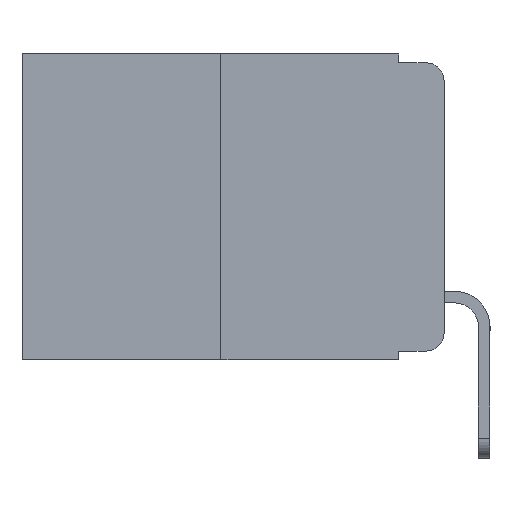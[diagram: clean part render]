
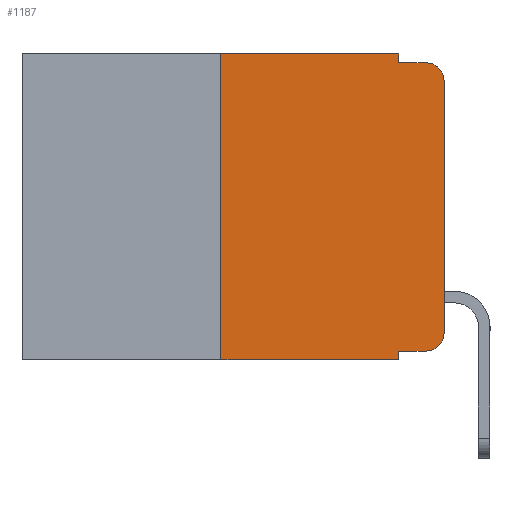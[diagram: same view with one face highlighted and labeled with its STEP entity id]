
A CAD part, left-side view. The second image highlights one B-rep face of the part: STEP entity #1187.
In plain terms, the highlighted planar face has unit normal (-1, 0, 0).
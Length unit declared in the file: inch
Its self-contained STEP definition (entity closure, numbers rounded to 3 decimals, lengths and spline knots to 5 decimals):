
#243 = ORIENTED_EDGE ( 'NONE', *, *, #24246, .T. ) ;
#959 = VERTEX_POINT ( 'NONE', #16289 ) ;
#1187 = ADVANCED_FACE ( 'NONE', ( #11730 ), #17278, .F. ) ;
#1302 = DIRECTION ( 'NONE',  ( 0., 0., -1. ) ) ;
#1364 = CARTESIAN_POINT ( 'NONE',  ( 0., 0., 0. ) ) ;
#1775 = CARTESIAN_POINT ( 'NONE',  ( 0., 0.051, 0. ) ) ;
#1872 = DIRECTION ( 'NONE',  ( 0., 0., -1. ) ) ;
#2029 = CARTESIAN_POINT ( 'NONE',  ( 0., 0.473, 0. ) ) ;
#2393 = ORIENTED_EDGE ( 'NONE', *, *, #10809, .F. ) ;
#2582 = ORIENTED_EDGE ( 'NONE', *, *, #19447, .F. ) ;
#2783 = LINE ( 'NONE', #19544, #12855 ) ;
#2857 = ORIENTED_EDGE ( 'NONE', *, *, #24707, .F. ) ;
#2881 = EDGE_CURVE ( 'NONE', #23649, #20933, #2783, .T. ) ;
#3012 = VERTEX_POINT ( 'NONE', #13358 ) ;
#3714 = VERTEX_POINT ( 'NONE', #15313 ) ;
#3827 = CARTESIAN_POINT ( 'NONE',  ( 0., 0.051, -0.333 ) ) ;
#4040 = CARTESIAN_POINT ( 'NONE',  ( 0., 0.051, -0.333 ) ) ;
#4198 = AXIS2_PLACEMENT_3D ( 'NONE', #2029, #18192, #18045 ) ;
#5019 = EDGE_CURVE ( 'NONE', #3714, #23166, #5313, .T. ) ;
#5313 = LINE ( 'NONE', #14935, #11199 ) ;
#6075 = EDGE_CURVE ( 'NONE', #959, #22323, #8268, .T. ) ;
#6189 = VERTEX_POINT ( 'NONE', #16887 ) ;
#6404 = VERTEX_POINT ( 'NONE', #3827 ) ;
#6521 = LINE ( 'NONE', #4040, #21585 ) ;
#6672 = CARTESIAN_POINT ( 'NONE',  ( 0., 0.051, 0. ) ) ;
#6964 = VERTEX_POINT ( 'NONE', #13438 ) ;
#7321 = AXIS2_PLACEMENT_3D ( 'NONE', #14525, #14499, #9034 ) ;
#7905 = ORIENTED_EDGE ( 'NONE', *, *, #24487, .T. ) ;
#8268 = CIRCLE ( 'NONE', #7321, 0.02 ) ;
#8710 = DIRECTION ( 'NONE',  ( 0., 0., -1. ) ) ;
#8722 = AXIS2_PLACEMENT_3D ( 'NONE', #24347, #13497, #1302 ) ;
#8977 = ORIENTED_EDGE ( 'NONE', *, *, #5019, .F. ) ;
#9034 = DIRECTION ( 'NONE',  ( 0., 0., -1. ) ) ;
#10068 = ORIENTED_EDGE ( 'NONE', *, *, #11366, .F. ) ;
#10809 = EDGE_CURVE ( 'NONE', #6404, #20933, #21530, .T. ) ;
#11160 = VECTOR ( 'NONE', #17271, 39.37008 ) ;
#11199 = VECTOR ( 'NONE', #20354, 39.37008 ) ;
#11221 = CARTESIAN_POINT ( 'NONE',  ( 0., 0.051, 0. ) ) ;
#11366 = EDGE_CURVE ( 'NONE', #23649, #3714, #21830, .T. ) ;
#11730 = FACE_OUTER_BOUND ( 'NONE', #18532, .T. ) ;
#11801 = LINE ( 'NONE', #1364, #11160 ) ;
#12694 = VECTOR ( 'NONE', #19967, 39.37008 ) ;
#12855 = VECTOR ( 'NONE', #18111, 39.37008 ) ;
#13014 = VECTOR ( 'NONE', #23698, 39.37008 ) ;
#13358 = CARTESIAN_POINT ( 'NONE',  ( 0., 0., -0.03 ) ) ;
#13438 = CARTESIAN_POINT ( 'NONE',  ( 0., 0.051, -0.01 ) ) ;
#13497 = DIRECTION ( 'NONE',  ( -1., 0., 0. ) ) ;
#13818 = ORIENTED_EDGE ( 'NONE', *, *, #18994, .T. ) ;
#14368 = ORIENTED_EDGE ( 'NONE', *, *, #6075, .T. ) ;
#14499 = DIRECTION ( 'NONE',  ( -1., 0., 0. ) ) ;
#14525 = CARTESIAN_POINT ( 'NONE',  ( 0., 0.02, -0.313 ) ) ;
#14935 = CARTESIAN_POINT ( 'NONE',  ( 0., 0.473, 0. ) ) ;
#15313 = CARTESIAN_POINT ( 'NONE',  ( 0., 0.25, 0. ) ) ;
#15994 = ORIENTED_EDGE ( 'NONE', *, *, #2881, .T. ) ;
#16289 = CARTESIAN_POINT ( 'NONE',  ( 0., 0.02, -0.333 ) ) ;
#16743 = VECTOR ( 'NONE', #1872, 39.37008 ) ;
#16887 = CARTESIAN_POINT ( 'NONE',  ( 0., 0.02, -0.01 ) ) ;
#17073 = VECTOR ( 'NONE', #8710, 39.37008 ) ;
#17271 = DIRECTION ( 'NONE',  ( 0., 0., 1. ) ) ;
#17278 = PLANE ( 'NONE',  #4198 ) ;
#18045 = DIRECTION ( 'NONE',  ( 0., 0., -1. ) ) ;
#18111 = DIRECTION ( 'NONE',  ( 0., -1., 0. ) ) ;
#18192 = DIRECTION ( 'NONE',  ( 1., 0., 0. ) ) ;
#18338 = CARTESIAN_POINT ( 'NONE',  ( 0., 0.051, -0.01 ) ) ;
#18532 = EDGE_LOOP ( 'NONE', ( #13818, #243, #2582, #2857, #8977, #10068, #15994, #2393, #7905, #14368 ) ) ;
#18994 = EDGE_CURVE ( 'NONE', #22323, #3012, #11801, .T. ) ;
#19435 = CARTESIAN_POINT ( 'NONE',  ( 0., 0.25, -0.343 ) ) ;
#19447 = EDGE_CURVE ( 'NONE', #6964, #6189, #23287, .T. ) ;
#19544 = CARTESIAN_POINT ( 'NONE',  ( 0., 0.473, -0.343 ) ) ;
#19650 = CIRCLE ( 'NONE', #8722, 0.02 ) ;
#19967 = DIRECTION ( 'NONE',  ( 0., 0., 1. ) ) ;
#20339 = CARTESIAN_POINT ( 'NONE',  ( 0., 0., -0.313 ) ) ;
#20354 = DIRECTION ( 'NONE',  ( 0., -1., 0. ) ) ;
#20933 = VERTEX_POINT ( 'NONE', #22441 ) ;
#21530 = LINE ( 'NONE', #1775, #16743 ) ;
#21585 = VECTOR ( 'NONE', #23035, 39.37008 ) ;
#21702 = CARTESIAN_POINT ( 'NONE',  ( 0., 0.25, 0. ) ) ;
#21830 = LINE ( 'NONE', #21702, #12694 ) ;
#22323 = VERTEX_POINT ( 'NONE', #20339 ) ;
#22441 = CARTESIAN_POINT ( 'NONE',  ( 0., 0.051, -0.343 ) ) ;
#22988 = LINE ( 'NONE', #6672, #17073 ) ;
#23035 = DIRECTION ( 'NONE',  ( 0., -1., 0. ) ) ;
#23166 = VERTEX_POINT ( 'NONE', #11221 ) ;
#23287 = LINE ( 'NONE', #18338, #13014 ) ;
#23649 = VERTEX_POINT ( 'NONE', #19435 ) ;
#23698 = DIRECTION ( 'NONE',  ( 0., -1., 0. ) ) ;
#24246 = EDGE_CURVE ( 'NONE', #3012, #6189, #19650, .T. ) ;
#24347 = CARTESIAN_POINT ( 'NONE',  ( 0., 0.02, -0.03 ) ) ;
#24487 = EDGE_CURVE ( 'NONE', #6404, #959, #6521, .T. ) ;
#24707 = EDGE_CURVE ( 'NONE', #23166, #6964, #22988, .T. ) ;
